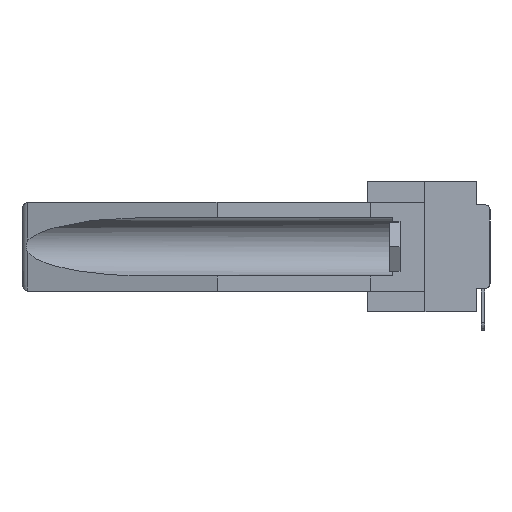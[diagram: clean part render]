
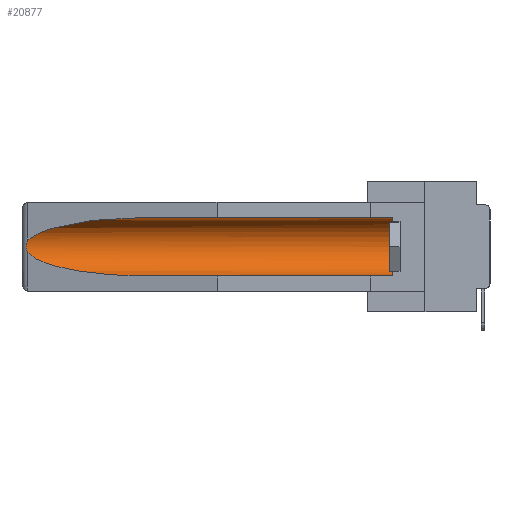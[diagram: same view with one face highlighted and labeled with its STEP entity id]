
A CAD part, left-side view. The second image highlights one B-rep face of the part: STEP entity #20877.
In plain terms, the highlighted cylindrical face has radius 2.857 mm (diameter 5.715 mm), a partial arc.
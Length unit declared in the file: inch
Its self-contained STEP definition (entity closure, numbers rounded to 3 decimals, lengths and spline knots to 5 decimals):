
#682 = ORIENTED_EDGE ( 'NONE', *, *, #27792, .T. ) ;
#1553 = VERTEX_POINT ( 'NONE', #13365 ) ;
#1573 = CYLINDRICAL_SURFACE ( 'NONE', #7833, 0.1125 ) ;
#2315 = CARTESIAN_POINT ( 'NONE',  ( 0.26597, 1.5296, -0.19026 ) ) ;
#2864 = ORIENTED_EDGE ( 'NONE', *, *, #17134, .T. ) ;
#3486 = CARTESIAN_POINT ( 'NONE',  ( 0.155, -0.30754, -0.1715 ) ) ;
#3637 = DIRECTION ( 'NONE',  ( 0., 0., 1. ) ) ;
#4507 = CARTESIAN_POINT ( 'NONE',  ( 0.26597, 1.52961, -0.15275 ) ) ;
#4836 =( BOUNDED_CURVE ( )  B_SPLINE_CURVE ( 3, ( #22576, #27980, #12355, #27432 ),
 .UNSPECIFIED., .F., .F. ) 
 B_SPLINE_CURVE_WITH_KNOTS ( ( 4, 4 ),
 ( 0.1948, 1.5708 ),
 .UNSPECIFIED. ) 
 CURVE ( )  GEOMETRIC_REPRESENTATION_ITEM ( )  RATIONAL_B_SPLINE_CURVE ( ( 1., 0.848, 0.848, 1. ) ) 
 REPRESENTATION_ITEM ( '' )  );
#5479 = VECTOR ( 'NONE', #7158, 39.37008 ) ;
#5654 = DIRECTION ( 'NONE',  ( 0., 1., 0. ) ) ;
#6598 = CARTESIAN_POINT ( 'NONE',  ( 0.2675, 1.53308, -0.16763 ) ) ;
#6858 = VERTEX_POINT ( 'NONE', #11889 ) ;
#7059 = CARTESIAN_POINT ( 'NONE',  ( 0.26537, 1.52718, -0.19328 ) ) ;
#7158 = DIRECTION ( 'NONE',  ( 0., 1., 0. ) ) ;
#7833 = AXIS2_PLACEMENT_3D ( 'NONE', #3486, #10559, #3637 ) ;
#8021 = CARTESIAN_POINT ( 'NONE',  ( 0.155, 1.07973, -0.059 ) ) ;
#8119 = VERTEX_POINT ( 'NONE', #18080 ) ;
#8289 = CARTESIAN_POINT ( 'NONE',  ( 0.21114, 1.30732, -0.059 ) ) ;
#8352 = VECTOR ( 'NONE', #5654, 39.37008 ) ;
#8519 = CARTESIAN_POINT ( 'NONE',  ( 0.26537, 1.52718, -0.19328 ) ) ;
#8796 = CARTESIAN_POINT ( 'NONE',  ( 0.26655, 1.53094, -0.18657 ) ) ;
#9630 = DIRECTION ( 'NONE',  ( 0., -1., 0. ) ) ;
#10559 = DIRECTION ( 'NONE',  ( 0., 1., 0. ) ) ;
#10720 = CARTESIAN_POINT ( 'NONE',  ( 0.2673, 1.5327, -0.16383 ) ) ;
#11295 = CARTESIAN_POINT ( 'NONE',  ( 0.155, -0.30754, -0.284 ) ) ;
#11302 = CARTESIAN_POINT ( 'NONE',  ( 0.2673, 1.53269, -0.17917 ) ) ;
#11383 = VERTEX_POINT ( 'NONE', #7059 ) ;
#11729 = EDGE_CURVE ( 'NONE', #11822, #18121, #19634, .T. ) ;
#11822 = VERTEX_POINT ( 'NONE', #20961 ) ;
#11889 = CARTESIAN_POINT ( 'NONE',  ( 0.155, 1.07973, -0.284 ) ) ;
#11900 = EDGE_CURVE ( 'NONE', #18121, #8119, #25701, .T. ) ;
#12153 = EDGE_LOOP ( 'NONE', ( #2864, #17399, #682, #26458, #21892, #27196 ) ) ;
#12355 = CARTESIAN_POINT ( 'NONE',  ( 0.21114, 1.30732, -0.284 ) ) ;
#12385 = CARTESIAN_POINT ( 'NONE',  ( 0.26537, 1.52718, -0.14972 ) ) ;
#13365 = CARTESIAN_POINT ( 'NONE',  ( 0.26537, 1.52718, -0.14972 ) ) ;
#13511 = CARTESIAN_POINT ( 'NONE',  ( 0.26654, 1.53092, -0.15636 ) ) ;
#13778 = DIRECTION ( 'NONE',  ( 0., 0., 1. ) ) ;
#13887 =( BOUNDED_CURVE ( )  B_SPLINE_CURVE ( 3, ( #8021, #8289, #26301, #12385 ),
 .UNSPECIFIED., .F., .F. ) 
 B_SPLINE_CURVE_WITH_KNOTS ( ( 4, 4 ),
 ( 4.71239, 6.08839 ),
 .UNSPECIFIED. ) 
 CURVE ( )  GEOMETRIC_REPRESENTATION_ITEM ( )  RATIONAL_B_SPLINE_CURVE ( ( 1., 0.848, 0.848, 1. ) ) 
 REPRESENTATION_ITEM ( '' )  );
#17134 = EDGE_CURVE ( 'NONE', #8119, #1553, #13887, .T. ) ;
#17399 = ORIENTED_EDGE ( 'NONE', *, *, #22430, .T. ) ;
#18080 = CARTESIAN_POINT ( 'NONE',  ( 0.155, 1.07973, -0.059 ) ) ;
#18121 = VERTEX_POINT ( 'NONE', #25133 ) ;
#19111 = FACE_OUTER_BOUND ( 'NONE', #12153, .T. ) ;
#19299 = EDGE_CURVE ( 'NONE', #11822, #6858, #27368, .T. ) ;
#19634 = CIRCLE ( 'NONE', #25302, 0.1125 ) ;
#20877 = ADVANCED_FACE ( 'NONE', ( #19111 ), #1573, .F. ) ;
#20961 = CARTESIAN_POINT ( 'NONE',  ( 0.155, 0.126, -0.284 ) ) ;
#21608 = B_SPLINE_CURVE_WITH_KNOTS ( 'NONE', 3,
 ( #26948, #4507, #13511, #10720, #6598, #26506, #11302, #8796, #2315, #8519 ),
 .UNSPECIFIED., .F., .F.,
 ( 4, 2, 2, 2, 4 ),
 ( 0., 0.00029, 0.00058, 0.00087, 0.00117 ),
 .UNSPECIFIED. ) ;
#21892 = ORIENTED_EDGE ( 'NONE', *, *, #11729, .T. ) ;
#22430 = EDGE_CURVE ( 'NONE', #1553, #11383, #21608, .T. ) ;
#22576 = CARTESIAN_POINT ( 'NONE',  ( 0.26537, 1.52718, -0.19328 ) ) ;
#25133 = CARTESIAN_POINT ( 'NONE',  ( 0.155, 0.126, -0.059 ) ) ;
#25302 = AXIS2_PLACEMENT_3D ( 'NONE', #25563, #9630, #13778 ) ;
#25563 = CARTESIAN_POINT ( 'NONE',  ( 0.155, 0.126, -0.1715 ) ) ;
#25701 = LINE ( 'NONE', #28493, #8352 ) ;
#26301 = CARTESIAN_POINT ( 'NONE',  ( 0.25451, 1.48313, -0.09465 ) ) ;
#26458 = ORIENTED_EDGE ( 'NONE', *, *, #19299, .F. ) ;
#26506 = CARTESIAN_POINT ( 'NONE',  ( 0.2675, 1.53308, -0.17534 ) ) ;
#26948 = CARTESIAN_POINT ( 'NONE',  ( 0.26537, 1.52718, -0.14972 ) ) ;
#27196 = ORIENTED_EDGE ( 'NONE', *, *, #11900, .T. ) ;
#27368 = LINE ( 'NONE', #11295, #5479 ) ;
#27432 = CARTESIAN_POINT ( 'NONE',  ( 0.155, 1.07973, -0.284 ) ) ;
#27792 = EDGE_CURVE ( 'NONE', #11383, #6858, #4836, .T. ) ;
#27980 = CARTESIAN_POINT ( 'NONE',  ( 0.25451, 1.48313, -0.24835 ) ) ;
#28493 = CARTESIAN_POINT ( 'NONE',  ( 0.155, -0.30754, -0.059 ) ) ;
